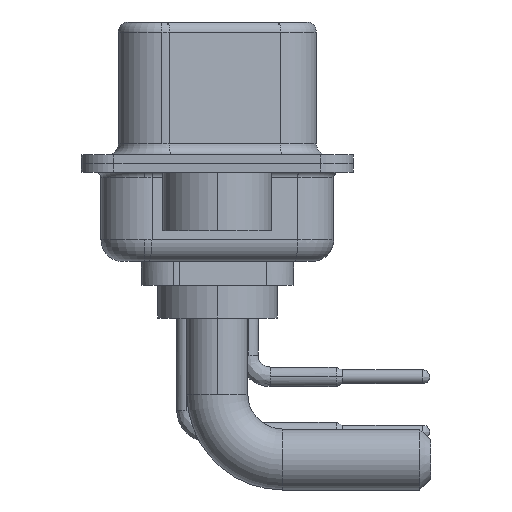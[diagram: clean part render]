
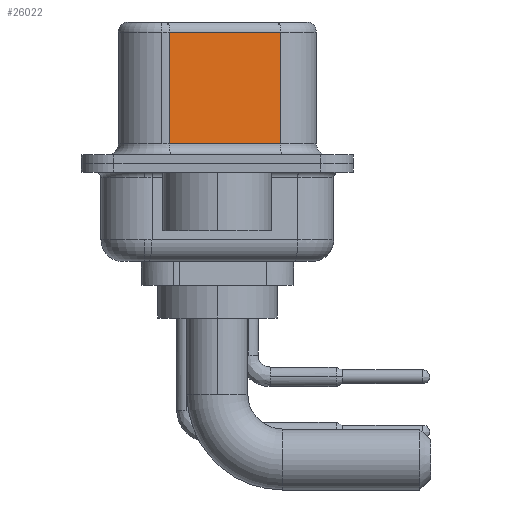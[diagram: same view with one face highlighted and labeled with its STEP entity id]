
A CAD part, left-side view. The second image highlights one B-rep face of the part: STEP entity #26022.
In plain terms, the highlighted planar face has unit normal (-0.985, -0.174, 0).
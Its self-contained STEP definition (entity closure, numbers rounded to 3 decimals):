
#156 = PLANE ( 'NONE',  #13109 ) ;
#2663 = CARTESIAN_POINT ( 'NONE',  ( 3.68, 2.203, 6.02 ) ) ;
#2679 = VECTOR ( 'NONE', #22905, 1000. ) ;
#3725 = VERTEX_POINT ( 'NONE', #2663 ) ;
#4272 = LINE ( 'NONE', #13138, #11877 ) ;
#4407 = EDGE_CURVE ( 'NONE', #12682, #24202, #4272, .T. ) ;
#4537 = CARTESIAN_POINT ( 'NONE',  ( 4.58, -2.897, 0.9 ) ) ;
#6292 = FACE_OUTER_BOUND ( 'NONE', #12769, .T. ) ;
#8280 = LINE ( 'NONE', #16547, #2679 ) ;
#8470 = CARTESIAN_POINT ( 'NONE',  ( 4.58, -2.897, 6.52 ) ) ;
#9785 = CARTESIAN_POINT ( 'NONE',  ( 4.58, -2.897, 6.52 ) ) ;
#9909 = LINE ( 'NONE', #9785, #16626 ) ;
#10108 = ORIENTED_EDGE ( 'NONE', *, *, #26545, .T. ) ;
#10221 = VERTEX_POINT ( 'NONE', #18816 ) ;
#11877 = VECTOR ( 'NONE', #23400, 1000. ) ;
#12682 = VERTEX_POINT ( 'NONE', #17275 ) ;
#12769 = EDGE_LOOP ( 'NONE', ( #18369, #20879, #10108, #22483 ) ) ;
#13109 = AXIS2_PLACEMENT_3D ( 'NONE', #8470, #26510, #14566 ) ;
#13138 = CARTESIAN_POINT ( 'NONE',  ( 4.58, -2.897, 0.9 ) ) ;
#14566 = DIRECTION ( 'NONE',  ( -0.174, 0.985, 0. ) ) ;
#16547 = CARTESIAN_POINT ( 'NONE',  ( 3.68, 2.203, 6.52 ) ) ;
#16626 = VECTOR ( 'NONE', #25769, 1000. ) ;
#17275 = CARTESIAN_POINT ( 'NONE',  ( 3.68, 2.203, 0.9 ) ) ;
#18200 = LINE ( 'NONE', #24582, #19935 ) ;
#18369 = ORIENTED_EDGE ( 'NONE', *, *, #21220, .F. ) ;
#18731 = DIRECTION ( 'NONE',  ( -0.174, 0.985, 0. ) ) ;
#18816 = CARTESIAN_POINT ( 'NONE',  ( 4.58, -2.897, 6.02 ) ) ;
#19935 = VECTOR ( 'NONE', #18731, 1000. ) ;
#20879 = ORIENTED_EDGE ( 'NONE', *, *, #23265, .T. ) ;
#21220 = EDGE_CURVE ( 'NONE', #10221, #24202, #9909, .T. ) ;
#22483 = ORIENTED_EDGE ( 'NONE', *, *, #4407, .T. ) ;
#22905 = DIRECTION ( 'NONE',  ( 0., 0., -1. ) ) ;
#23265 = EDGE_CURVE ( 'NONE', #10221, #3725, #18200, .T. ) ;
#23400 = DIRECTION ( 'NONE',  ( 0.174, -0.985, 0. ) ) ;
#24202 = VERTEX_POINT ( 'NONE', #4537 ) ;
#24582 = CARTESIAN_POINT ( 'NONE',  ( 4.58, -2.897, 6.02 ) ) ;
#25769 = DIRECTION ( 'NONE',  ( 0., 0., -1. ) ) ;
#26022 = ADVANCED_FACE ( 'NONE', ( #6292 ), #156, .F. ) ;
#26510 = DIRECTION ( 'NONE',  ( 0.985, 0.174, 0. ) ) ;
#26545 = EDGE_CURVE ( 'NONE', #3725, #12682, #8280, .T. ) ;
